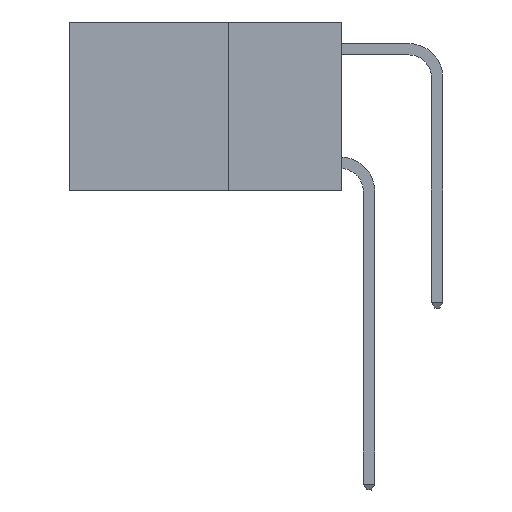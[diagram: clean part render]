
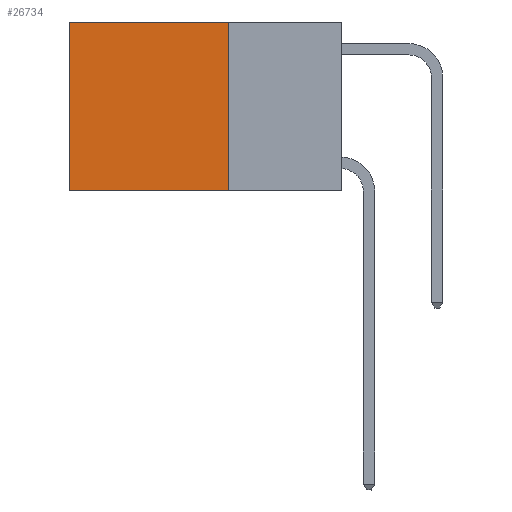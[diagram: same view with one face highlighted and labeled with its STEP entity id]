
A CAD part, left-side view. The second image highlights one B-rep face of the part: STEP entity #26734.
In plain terms, the highlighted planar face has unit normal (-1, 0, 0).
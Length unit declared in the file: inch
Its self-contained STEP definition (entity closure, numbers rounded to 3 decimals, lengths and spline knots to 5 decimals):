
#502 = VERTEX_POINT ( 'NONE', #21693 ) ;
#2153 = DIRECTION ( 'NONE',  ( 0., 0., -1. ) ) ;
#2868 = ORIENTED_EDGE ( 'NONE', *, *, #28031, .F. ) ;
#2981 = ORIENTED_EDGE ( 'NONE', *, *, #18750, .F. ) ;
#3015 = VERTEX_POINT ( 'NONE', #21169 ) ;
#3250 = CARTESIAN_POINT ( 'NONE',  ( 0.2625, 0.6, 0. ) ) ;
#6106 = DIRECTION ( 'NONE',  ( 1., 0., 0. ) ) ;
#6407 = VECTOR ( 'NONE', #10093, 39.37008 ) ;
#6609 = ORIENTED_EDGE ( 'NONE', *, *, #7145, .T. ) ;
#7145 = EDGE_CURVE ( 'NONE', #3015, #502, #7980, .T. ) ;
#7297 = CARTESIAN_POINT ( 'NONE',  ( 0.2625, 0.25, -0.37 ) ) ;
#7980 = LINE ( 'NONE', #8109, #6407 ) ;
#8109 = CARTESIAN_POINT ( 'NONE',  ( 0.2625, 0.25, 0. ) ) ;
#9128 = LINE ( 'NONE', #7297, #19533 ) ;
#10093 = DIRECTION ( 'NONE',  ( 0., 1., 0. ) ) ;
#11813 = DIRECTION ( 'NONE',  ( 0., 1., 0. ) ) ;
#12483 = ORIENTED_EDGE ( 'NONE', *, *, #12928, .T. ) ;
#12928 = EDGE_CURVE ( 'NONE', #502, #13704, #27435, .T. ) ;
#13704 = VERTEX_POINT ( 'NONE', #24400 ) ;
#13925 = FACE_OUTER_BOUND ( 'NONE', #24978, .T. ) ;
#14173 = DIRECTION ( 'NONE',  ( 0., 0., -1. ) ) ;
#16567 = VECTOR ( 'NONE', #14173, 39.37008 ) ;
#18750 = EDGE_CURVE ( 'NONE', #3015, #21348, #26196, .T. ) ;
#19314 = DIRECTION ( 'NONE',  ( 0., 0., -1. ) ) ;
#19527 = CARTESIAN_POINT ( 'NONE',  ( 0.2625, 0.25, -0.37 ) ) ;
#19533 = VECTOR ( 'NONE', #11813, 39.37008 ) ;
#20465 = CARTESIAN_POINT ( 'NONE',  ( 0.2625, 0.25, 0. ) ) ;
#21083 = VECTOR ( 'NONE', #2153, 39.37008 ) ;
#21169 = CARTESIAN_POINT ( 'NONE',  ( 0.2625, 0.25, 0. ) ) ;
#21348 = VERTEX_POINT ( 'NONE', #19527 ) ;
#21693 = CARTESIAN_POINT ( 'NONE',  ( 0.2625, 0.6, 0. ) ) ;
#21812 = AXIS2_PLACEMENT_3D ( 'NONE', #20465, #6106, #19314 ) ;
#22612 = PLANE ( 'NONE',  #21812 ) ;
#23786 = CARTESIAN_POINT ( 'NONE',  ( 0.2625, 0.25, 0. ) ) ;
#24400 = CARTESIAN_POINT ( 'NONE',  ( 0.2625, 0.6, -0.37 ) ) ;
#24978 = EDGE_LOOP ( 'NONE', ( #12483, #2868, #2981, #6609 ) ) ;
#26196 = LINE ( 'NONE', #23786, #21083 ) ;
#26734 = ADVANCED_FACE ( 'NONE', ( #13925 ), #22612, .F. ) ;
#27435 = LINE ( 'NONE', #3250, #16567 ) ;
#28031 = EDGE_CURVE ( 'NONE', #21348, #13704, #9128, .T. ) ;
